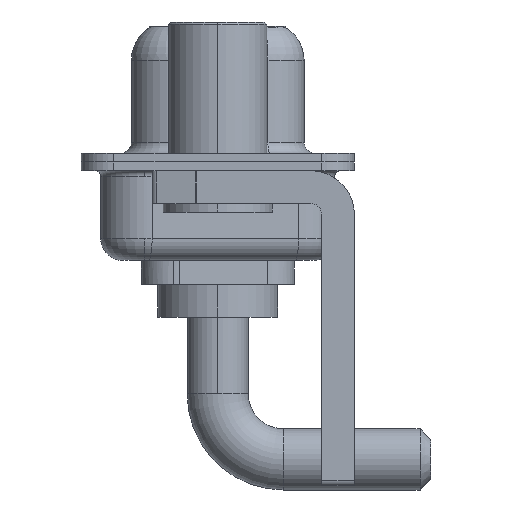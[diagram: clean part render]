
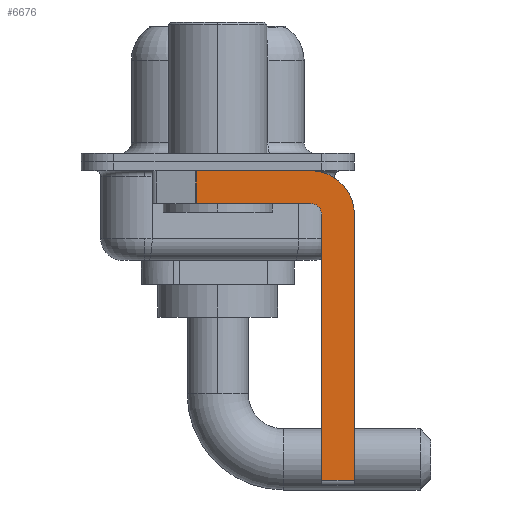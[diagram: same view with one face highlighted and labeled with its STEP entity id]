
A CAD part, left-side view. The second image highlights one B-rep face of the part: STEP entity #6676.
In plain terms, the highlighted planar face has unit normal (-1, 0, 0).
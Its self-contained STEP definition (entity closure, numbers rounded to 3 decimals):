
#60 = ORIENTED_EDGE ( 'NONE', *, *, #2089, .T. ) ;
#253 = VERTEX_POINT ( 'NONE', #9594 ) ;
#417 = CARTESIAN_POINT ( 'NONE',  ( -2.9, -4.75, -2.4 ) ) ;
#466 = CARTESIAN_POINT ( 'NONE',  ( -2.9, 0.978, -1.9 ) ) ;
#678 = DIRECTION ( 'NONE',  ( 0., 0., -1. ) ) ;
#826 = AXIS2_PLACEMENT_3D ( 'NONE', #14103, #3388, #1158 ) ;
#971 = ORIENTED_EDGE ( 'NONE', *, *, #4863, .F. ) ;
#1011 = DIRECTION ( 'NONE',  ( 0., 0., 1. ) ) ;
#1120 = CARTESIAN_POINT ( 'NONE',  ( -2.9, -4.25, -0.4 ) ) ;
#1158 = DIRECTION ( 'NONE',  ( 0., 0., -1. ) ) ;
#1990 = CARTESIAN_POINT ( 'NONE',  ( -2.9, -4.25, -1.9 ) ) ;
#2022 = VECTOR ( 'NONE', #11377, 1000. ) ;
#2061 = PLANE ( 'NONE',  #6086 ) ;
#2089 = EDGE_CURVE ( 'NONE', #253, #12130, #6563, .T. ) ;
#2749 = ORIENTED_EDGE ( 'NONE', *, *, #14602, .F. ) ;
#2903 = ORIENTED_EDGE ( 'NONE', *, *, #12493, .T. ) ;
#3160 = EDGE_CURVE ( 'NONE', #4369, #11679, #7945, .T. ) ;
#3388 = DIRECTION ( 'NONE',  ( 1., 0., 0. ) ) ;
#3493 = DIRECTION ( 'NONE',  ( 0., -1., 0. ) ) ;
#3685 = CARTESIAN_POINT ( 'NONE',  ( -2.9, 0.978, -1.9 ) ) ;
#4035 = DIRECTION ( 'NONE',  ( 0., -1., 0. ) ) ;
#4369 = VERTEX_POINT ( 'NONE', #1120 ) ;
#4464 = VERTEX_POINT ( 'NONE', #12897 ) ;
#4863 = EDGE_CURVE ( 'NONE', #4464, #4369, #5730, .T. ) ;
#5189 = DIRECTION ( 'NONE',  ( 0., 0., -1. ) ) ;
#5263 = LINE ( 'NONE', #466, #10289 ) ;
#5274 = VECTOR ( 'NONE', #678, 1000. ) ;
#5605 = EDGE_CURVE ( 'NONE', #253, #11582, #14952, .T. ) ;
#5675 = EDGE_LOOP ( 'NONE', ( #971, #2903, #13328, #2749, #5747, #60, #7632, #8072 ) ) ;
#5730 = LINE ( 'NONE', #10488, #6556 ) ;
#5747 = ORIENTED_EDGE ( 'NONE', *, *, #5605, .F. ) ;
#5756 = DIRECTION ( 'NONE',  ( 1., 0., 0. ) ) ;
#6086 = AXIS2_PLACEMENT_3D ( 'NONE', #12744, #5756, #8986 ) ;
#6556 = VECTOR ( 'NONE', #3493, 1000. ) ;
#6563 = LINE ( 'NONE', #14873, #8492 ) ;
#6676 = ADVANCED_FACE ( 'NONE', ( #13911 ), #2061, .F. ) ;
#7632 = ORIENTED_EDGE ( 'NONE', *, *, #11179, .F. ) ;
#7782 = VECTOR ( 'NONE', #1011, 1000. ) ;
#7945 = CIRCLE ( 'NONE', #826, 2. ) ;
#8010 = CARTESIAN_POINT ( 'NONE',  ( -2.9, -4.75, -14.8 ) ) ;
#8072 = ORIENTED_EDGE ( 'NONE', *, *, #3160, .F. ) ;
#8158 = VERTEX_POINT ( 'NONE', #10436 ) ;
#8492 = VECTOR ( 'NONE', #4035, 1000. ) ;
#8986 = DIRECTION ( 'NONE',  ( 0., 0., -1. ) ) ;
#9276 = LINE ( 'NONE', #1990, #2022 ) ;
#9556 = DIRECTION ( 'NONE',  ( -1., 0., 0. ) ) ;
#9594 = CARTESIAN_POINT ( 'NONE',  ( -2.9, -4.75, -14.55 ) ) ;
#10037 = EDGE_CURVE ( 'NONE', #8158, #12731, #9276, .T. ) ;
#10087 = CIRCLE ( 'NONE', #12057, 0.5 ) ;
#10141 = LINE ( 'NONE', #13697, #5274 ) ;
#10289 = VECTOR ( 'NONE', #5189, 1000. ) ;
#10436 = CARTESIAN_POINT ( 'NONE',  ( -2.9, -4.25, -1.9 ) ) ;
#10488 = CARTESIAN_POINT ( 'NONE',  ( -2.9, 3., -0.4 ) ) ;
#11179 = EDGE_CURVE ( 'NONE', #11679, #12130, #10141, .T. ) ;
#11377 = DIRECTION ( 'NONE',  ( 0., 1., 0. ) ) ;
#11582 = VERTEX_POINT ( 'NONE', #417 ) ;
#11679 = VERTEX_POINT ( 'NONE', #14902 ) ;
#12019 = DIRECTION ( 'NONE',  ( 0., 0., 1. ) ) ;
#12057 = AXIS2_PLACEMENT_3D ( 'NONE', #13189, #9556, #12019 ) ;
#12130 = VERTEX_POINT ( 'NONE', #13660 ) ;
#12493 = EDGE_CURVE ( 'NONE', #4464, #12731, #5263, .T. ) ;
#12731 = VERTEX_POINT ( 'NONE', #3685 ) ;
#12744 = CARTESIAN_POINT ( 'NONE',  ( -2.9, -4.25, -2.4 ) ) ;
#12897 = CARTESIAN_POINT ( 'NONE',  ( -2.9, 0.978, -0.4 ) ) ;
#13189 = CARTESIAN_POINT ( 'NONE',  ( -2.9, -4.25, -2.4 ) ) ;
#13328 = ORIENTED_EDGE ( 'NONE', *, *, #10037, .F. ) ;
#13660 = CARTESIAN_POINT ( 'NONE',  ( -2.9, -6.25, -14.55 ) ) ;
#13697 = CARTESIAN_POINT ( 'NONE',  ( -2.9, -6.25, -2.4 ) ) ;
#13911 = FACE_OUTER_BOUND ( 'NONE', #5675, .T. ) ;
#14103 = CARTESIAN_POINT ( 'NONE',  ( -2.9, -4.25, -2.4 ) ) ;
#14602 = EDGE_CURVE ( 'NONE', #11582, #8158, #10087, .T. ) ;
#14873 = CARTESIAN_POINT ( 'NONE',  ( -2.9, -4.25, -14.55 ) ) ;
#14902 = CARTESIAN_POINT ( 'NONE',  ( -2.9, -6.25, -2.4 ) ) ;
#14952 = LINE ( 'NONE', #8010, #7782 ) ;
